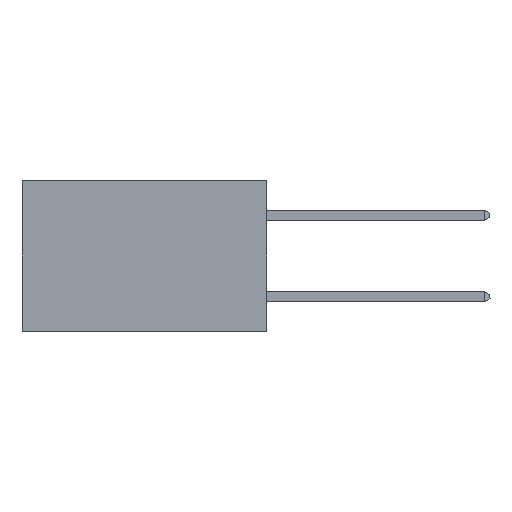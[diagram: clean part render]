
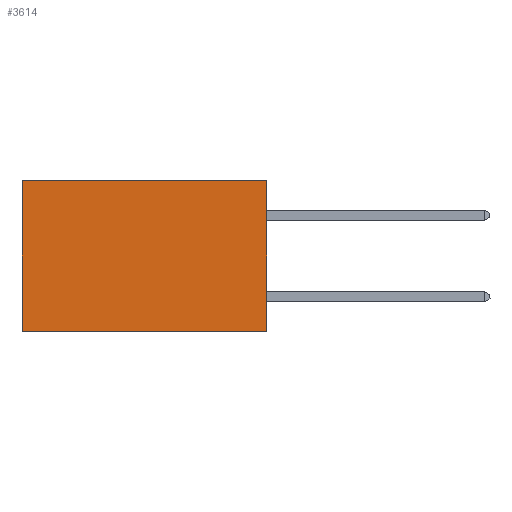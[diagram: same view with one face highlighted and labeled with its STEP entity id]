
A CAD part, left-side view. The second image highlights one B-rep face of the part: STEP entity #3614.
In plain terms, the highlighted planar face has unit normal (-1, 0, 0).
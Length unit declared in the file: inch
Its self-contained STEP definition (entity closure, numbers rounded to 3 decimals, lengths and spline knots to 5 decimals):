
#419 = VERTEX_POINT ( 'NONE', #4122 ) ;
#597 = DIRECTION ( 'NONE',  ( 0., 1., 0. ) ) ;
#760 = PLANE ( 'NONE',  #5148 ) ;
#907 = EDGE_CURVE ( 'NONE', #5510, #1325, #1871, .T. ) ;
#1325 = VERTEX_POINT ( 'NONE', #4844 ) ;
#1871 = LINE ( 'NONE', #8795, #6488 ) ;
#2107 = DIRECTION ( 'NONE',  ( 0., 1., 0. ) ) ;
#2177 = VECTOR ( 'NONE', #2107, 39.37008 ) ;
#2206 = DIRECTION ( 'NONE',  ( 0., 0., -1. ) ) ;
#2543 = CARTESIAN_POINT ( 'NONE',  ( 0.2875, 0., -0.37 ) ) ;
#2688 = EDGE_CURVE ( 'NONE', #419, #5510, #3856, .T. ) ;
#3081 = EDGE_CURVE ( 'NONE', #4470, #1325, #7435, .T. ) ;
#3241 = ORIENTED_EDGE ( 'NONE', *, *, #907, .F. ) ;
#3518 = DIRECTION ( 'NONE',  ( 1., 0., 0. ) ) ;
#3614 = ADVANCED_FACE ( 'NONE', ( #8419 ), #760, .F. ) ;
#3856 = LINE ( 'NONE', #11510, #9279 ) ;
#3891 = CARTESIAN_POINT ( 'NONE',  ( 0.2875, 0., 0. ) ) ;
#4122 = CARTESIAN_POINT ( 'NONE',  ( 0.2875, 0., 0. ) ) ;
#4470 = VERTEX_POINT ( 'NONE', #11236 ) ;
#4611 = EDGE_LOOP ( 'NONE', ( #5623, #3241, #8033, #8605 ) ) ;
#4844 = CARTESIAN_POINT ( 'NONE',  ( 0.2875, 0.6, -0.37 ) ) ;
#5148 = AXIS2_PLACEMENT_3D ( 'NONE', #11892, #3518, #6388 ) ;
#5510 = VERTEX_POINT ( 'NONE', #2543 ) ;
#5623 = ORIENTED_EDGE ( 'NONE', *, *, #3081, .T. ) ;
#6388 = DIRECTION ( 'NONE',  ( 0., 0., -1. ) ) ;
#6488 = VECTOR ( 'NONE', #597, 39.37008 ) ;
#6506 = DIRECTION ( 'NONE',  ( 0., 0., -1. ) ) ;
#7148 = EDGE_CURVE ( 'NONE', #419, #4470, #9639, .T. ) ;
#7435 = LINE ( 'NONE', #7638, #8977 ) ;
#7638 = CARTESIAN_POINT ( 'NONE',  ( 0.2875, 0.6, 0. ) ) ;
#8033 = ORIENTED_EDGE ( 'NONE', *, *, #2688, .F. ) ;
#8419 = FACE_OUTER_BOUND ( 'NONE', #4611, .T. ) ;
#8605 = ORIENTED_EDGE ( 'NONE', *, *, #7148, .T. ) ;
#8795 = CARTESIAN_POINT ( 'NONE',  ( 0.2875, 0., -0.37 ) ) ;
#8977 = VECTOR ( 'NONE', #2206, 39.37008 ) ;
#9279 = VECTOR ( 'NONE', #6506, 39.37008 ) ;
#9639 = LINE ( 'NONE', #3891, #2177 ) ;
#11236 = CARTESIAN_POINT ( 'NONE',  ( 0.2875, 0.6, 0. ) ) ;
#11510 = CARTESIAN_POINT ( 'NONE',  ( 0.2875, 0., 0. ) ) ;
#11892 = CARTESIAN_POINT ( 'NONE',  ( 0.2875, 0., 0. ) ) ;
